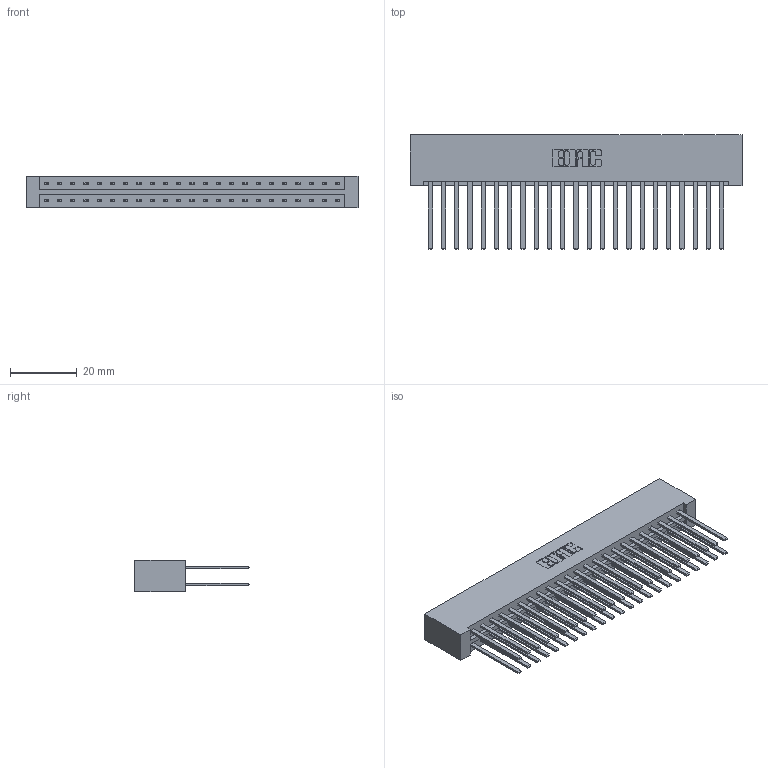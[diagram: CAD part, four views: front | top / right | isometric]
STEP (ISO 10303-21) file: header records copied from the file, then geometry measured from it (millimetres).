
FILE_DESCRIPTION (( 'STEP AP203' ), '1' );
FILE_NAME ('833-046-544-201.STEP', '2020-06-04T14:36:46', ( '' ), ( '' ), 'SwSTEP 2.0', 'SolidWorks 2020', '' );
FILE_SCHEMA (( 'CONFIG_CONTROL_DESIGN' ));
Length unit declared in the file: inch
Products named in the file (3): 833-046-544-201; 345-292-001_345-293-144; 833 Part_Lugless
Assembly tree (47 placements, depth 2):
  833-046-544-201
    833 Part_Lugless
    345-292-001_345-293-144  x46
Bounding box: 99.39 x 34.3 x 9.4 mm (x, y, z)
Volume: 11246.5 mm3; surface area: 15192.6 mm2
Topology: 47 solids, 47 shells, 2222 faces, 6589 edges, 4330 vertices
Faces by surface type: plane 1538, cylinder 684
Entity records: 16793 total; most frequent: CARTESIAN_POINT 2802, ORIENTED_EDGE 2738, DIRECTION 2417, EDGE_CURVE 1369, LINE 1253, VECTOR 1253, VERTEX_POINT 910, AXIS2_PLACEMENT_3D 582
